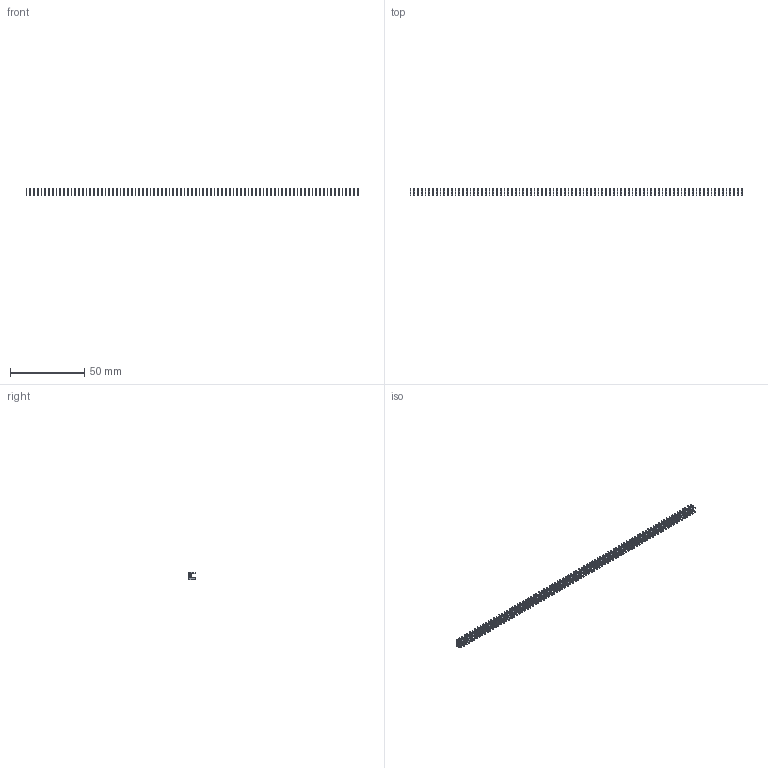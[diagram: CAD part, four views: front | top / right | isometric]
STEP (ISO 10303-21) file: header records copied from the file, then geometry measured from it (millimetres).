
FILE_DESCRIPTION (( 'STEP AP203' ), '1' );
FILE_NAME ('105-089-208-100.STEP', '2020-04-08T01:12:10', ( '' ), ( '' ), 'SwSTEP 2.0', 'SolidWorks 2016', '' );
FILE_SCHEMA (( 'CONFIG_CONTROL_DESIGN' ));
Length unit declared in the file: inch
Products named in the file (2): 105-089-208-100; 100-290-001_100-290-208
Assembly tree (89 placements, depth 2):
  105-089-208-100
    100-290-001_100-290-208  x89
Bounding box: 224.03 x 4.83 x 5.17 mm (x, y, z)
Volume: 612.4 mm3; surface area: 3782.1 mm2
Topology: 89 solids, 89 shells, 2225 faces, 6141 edges, 4094 vertices
Faces by surface type: plane 1958, cylinder 267
Entity records: 3805 total; most frequent: DIRECTION 309, CARTESIAN_POINT 232, COORDINATED_UNIVERSAL_TIME_OFFSET 188, DATE_AND_TIME 188, LOCAL_TIME 188, CALENDAR_DATE 188, ORIENTED_EDGE 138, AXIS2_PLACEMENT_3D 123
